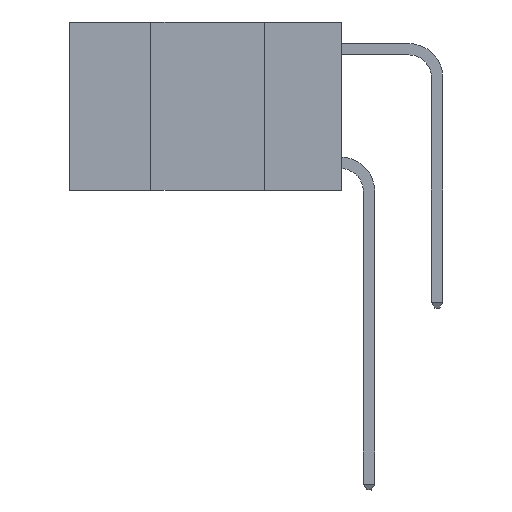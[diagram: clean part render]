
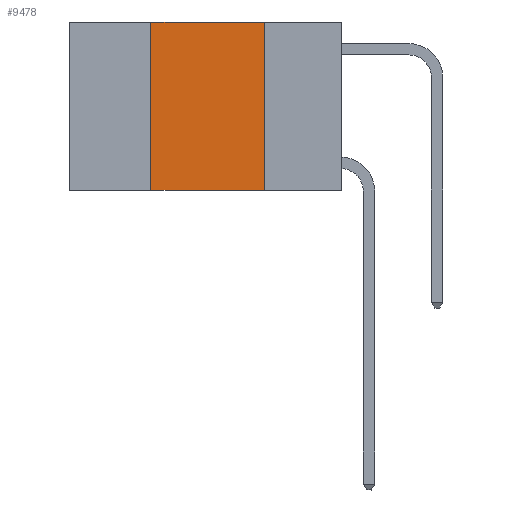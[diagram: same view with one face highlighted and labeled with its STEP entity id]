
A CAD part, left-side view. The second image highlights one B-rep face of the part: STEP entity #9478.
In plain terms, the highlighted planar face has unit normal (-1, 0, 0).
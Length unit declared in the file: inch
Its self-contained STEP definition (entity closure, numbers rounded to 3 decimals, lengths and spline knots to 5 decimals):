
#80 = VERTEX_POINT ( 'NONE', #1377 ) ;
#1377 = CARTESIAN_POINT ( 'NONE',  ( 0., 0.17, 0. ) ) ;
#1437 = DIRECTION ( 'NONE',  ( 0., -1., 0. ) ) ;
#1692 = DIRECTION ( 'NONE',  ( 1., 0., 0. ) ) ;
#1711 = LINE ( 'NONE', #6107, #6464 ) ;
#1827 = CARTESIAN_POINT ( 'NONE',  ( 0., 0.17, 0. ) ) ;
#1839 = FACE_OUTER_BOUND ( 'NONE', #6443, .T. ) ;
#1945 = EDGE_CURVE ( 'NONE', #9766, #80, #13255, .T. ) ;
#2110 = LINE ( 'NONE', #4342, #9203 ) ;
#3166 = CARTESIAN_POINT ( 'NONE',  ( 0., 0.17, -0.37 ) ) ;
#4342 = CARTESIAN_POINT ( 'NONE',  ( 0., 0.42, 0. ) ) ;
#4769 = AXIS2_PLACEMENT_3D ( 'NONE', #11106, #1692, #5530 ) ;
#5105 = ORIENTED_EDGE ( 'NONE', *, *, #8647, .F. ) ;
#5228 = VERTEX_POINT ( 'NONE', #10047 ) ;
#5530 = DIRECTION ( 'NONE',  ( 0., 0., -1. ) ) ;
#6107 = CARTESIAN_POINT ( 'NONE',  ( 0., 0.6, -0.37 ) ) ;
#6443 = EDGE_LOOP ( 'NONE', ( #10153, #14406, #5105, #8394 ) ) ;
#6464 = VECTOR ( 'NONE', #12061, 39.37008 ) ;
#7840 = VECTOR ( 'NONE', #14966, 39.37008 ) ;
#8394 = ORIENTED_EDGE ( 'NONE', *, *, #8821, .T. ) ;
#8550 = CARTESIAN_POINT ( 'NONE',  ( 0., 0.42, 0. ) ) ;
#8647 = EDGE_CURVE ( 'NONE', #5228, #9766, #2110, .T. ) ;
#8821 = EDGE_CURVE ( 'NONE', #5228, #14197, #1711, .T. ) ;
#8822 = DIRECTION ( 'NONE',  ( 0., 0., 1. ) ) ;
#9014 = LINE ( 'NONE', #1827, #7840 ) ;
#9203 = VECTOR ( 'NONE', #8822, 39.37008 ) ;
#9478 = ADVANCED_FACE ( 'NONE', ( #1839 ), #14678, .F. ) ;
#9766 = VERTEX_POINT ( 'NONE', #8550 ) ;
#10047 = CARTESIAN_POINT ( 'NONE',  ( 0., 0.42, -0.37 ) ) ;
#10153 = ORIENTED_EDGE ( 'NONE', *, *, #11245, .F. ) ;
#11106 = CARTESIAN_POINT ( 'NONE',  ( 0., 0.6, 0. ) ) ;
#11245 = EDGE_CURVE ( 'NONE', #80, #14197, #9014, .T. ) ;
#12061 = DIRECTION ( 'NONE',  ( 0., -1., 0. ) ) ;
#13255 = LINE ( 'NONE', #14491, #15260 ) ;
#14197 = VERTEX_POINT ( 'NONE', #3166 ) ;
#14406 = ORIENTED_EDGE ( 'NONE', *, *, #1945, .F. ) ;
#14491 = CARTESIAN_POINT ( 'NONE',  ( 0., 0.6, 0. ) ) ;
#14678 = PLANE ( 'NONE',  #4769 ) ;
#14966 = DIRECTION ( 'NONE',  ( 0., 0., -1. ) ) ;
#15260 = VECTOR ( 'NONE', #1437, 39.37008 ) ;
